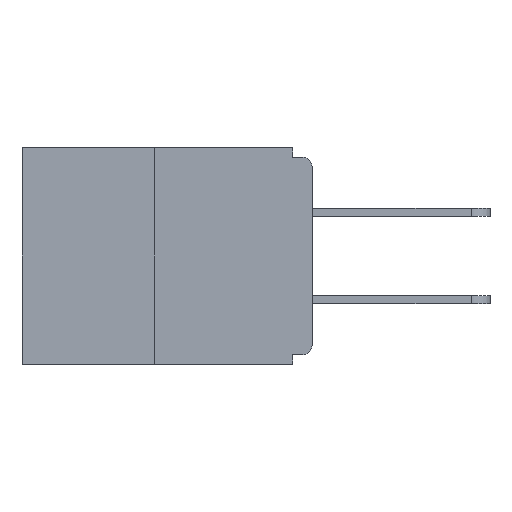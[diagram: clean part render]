
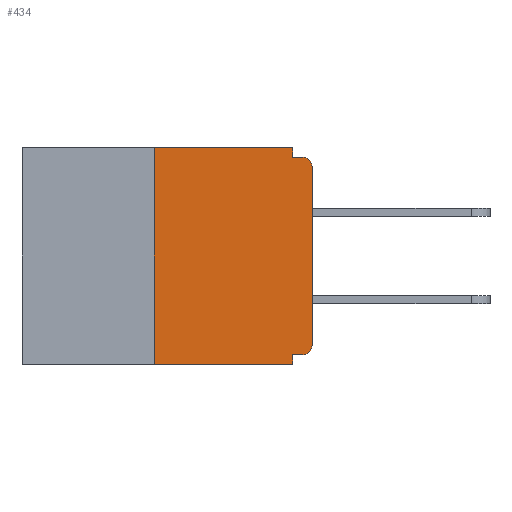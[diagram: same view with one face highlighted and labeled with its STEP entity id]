
A CAD part, left-side view. The second image highlights one B-rep face of the part: STEP entity #434.
In plain terms, the highlighted planar face has unit normal (-1, 0, 0).
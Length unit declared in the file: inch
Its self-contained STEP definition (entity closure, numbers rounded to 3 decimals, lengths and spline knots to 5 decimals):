
#392 = CARTESIAN_POINT ( 'NONE',  ( 0., 0.015, -0.015 ) ) ;
#434 = ADVANCED_FACE ( 'NONE', ( #11077 ), #12126, .F. ) ;
#516 = CARTESIAN_POINT ( 'NONE',  ( 0., 0.46, -0.343 ) ) ;
#550 = DIRECTION ( 'NONE',  ( -1., 0., 0. ) ) ;
#561 = CARTESIAN_POINT ( 'NONE',  ( 0., 0., -0.313 ) ) ;
#722 = CARTESIAN_POINT ( 'NONE',  ( 0., 0., -0.328 ) ) ;
#822 = VERTEX_POINT ( 'NONE', #561 ) ;
#909 = EDGE_CURVE ( 'NONE', #7638, #8690, #3916, .T. ) ;
#922 = CARTESIAN_POINT ( 'NONE',  ( 0., 0., -0.03 ) ) ;
#1101 = CARTESIAN_POINT ( 'NONE',  ( 0., 0.015, -0.328 ) ) ;
#1700 = EDGE_CURVE ( 'NONE', #7556, #10894, #4006, .T. ) ;
#1918 = VERTEX_POINT ( 'NONE', #5938 ) ;
#2105 = EDGE_CURVE ( 'NONE', #7172, #822, #6820, .T. ) ;
#2283 = ORIENTED_EDGE ( 'NONE', *, *, #9506, .F. ) ;
#2381 = ORIENTED_EDGE ( 'NONE', *, *, #909, .F. ) ;
#2509 = EDGE_CURVE ( 'NONE', #10184, #7638, #7995, .T. ) ;
#2531 = CARTESIAN_POINT ( 'NONE',  ( 0., 0.031, -0.343 ) ) ;
#2669 = DIRECTION ( 'NONE',  ( 0., 1., 0. ) ) ;
#2683 = VERTEX_POINT ( 'NONE', #4005 ) ;
#2718 = DIRECTION ( 'NONE',  ( 0., 0., -1. ) ) ;
#2997 = CARTESIAN_POINT ( 'NONE',  ( 0., 0.25, 0. ) ) ;
#3436 = VECTOR ( 'NONE', #7219, 39.37008 ) ;
#3525 = DIRECTION ( 'NONE',  ( 0., 0., 1. ) ) ;
#3538 = LINE ( 'NONE', #2531, #10818 ) ;
#3569 = DIRECTION ( 'NONE',  ( 0., 0., -1. ) ) ;
#3680 = CARTESIAN_POINT ( 'NONE',  ( 0., 0., -0.015 ) ) ;
#3856 = VECTOR ( 'NONE', #3525, 39.37008 ) ;
#3916 = LINE ( 'NONE', #8224, #10313 ) ;
#3985 = LINE ( 'NONE', #8047, #5644 ) ;
#4005 = CARTESIAN_POINT ( 'NONE',  ( 0., 0.031, -0.015 ) ) ;
#4006 = CIRCLE ( 'NONE', #6271, 0.015 ) ;
#4394 = EDGE_CURVE ( 'NONE', #10184, #8232, #5365, .T. ) ;
#4419 = DIRECTION ( 'NONE',  ( 0., -1., 0. ) ) ;
#4447 = EDGE_CURVE ( 'NONE', #7172, #1918, #9519, .T. ) ;
#4490 = DIRECTION ( 'NONE',  ( 0., 0., 1. ) ) ;
#4740 = LINE ( 'NONE', #8037, #12024 ) ;
#4776 = AXIS2_PLACEMENT_3D ( 'NONE', #8966, #550, #9967 ) ;
#4802 = ORIENTED_EDGE ( 'NONE', *, *, #7922, .F. ) ;
#5168 = VECTOR ( 'NONE', #6536, 39.37008 ) ;
#5365 = LINE ( 'NONE', #516, #3436 ) ;
#5521 = DIRECTION ( 'NONE',  ( 1., 0., 0. ) ) ;
#5644 = VECTOR ( 'NONE', #4490, 39.37008 ) ;
#5917 = LINE ( 'NONE', #3680, #5168 ) ;
#5933 = EDGE_CURVE ( 'NONE', #822, #7556, #3985, .T. ) ;
#5938 = CARTESIAN_POINT ( 'NONE',  ( 0., 0.031, -0.328 ) ) ;
#6271 = AXIS2_PLACEMENT_3D ( 'NONE', #7486, #12161, #2718 ) ;
#6536 = DIRECTION ( 'NONE',  ( 0., -1., 0. ) ) ;
#6820 = CIRCLE ( 'NONE', #4776, 0.015 ) ;
#7172 = VERTEX_POINT ( 'NONE', #1101 ) ;
#7200 = DIRECTION ( 'NONE',  ( 0., 0., -1. ) ) ;
#7219 = DIRECTION ( 'NONE',  ( 0., -1., 0. ) ) ;
#7486 = CARTESIAN_POINT ( 'NONE',  ( 0., 0.015, -0.03 ) ) ;
#7556 = VERTEX_POINT ( 'NONE', #922 ) ;
#7638 = VERTEX_POINT ( 'NONE', #2997 ) ;
#7922 = EDGE_CURVE ( 'NONE', #2683, #10894, #5917, .T. ) ;
#7995 = LINE ( 'NONE', #11175, #3856 ) ;
#8037 = CARTESIAN_POINT ( 'NONE',  ( 0., 0.031, 0. ) ) ;
#8047 = CARTESIAN_POINT ( 'NONE',  ( 0., 0., 0. ) ) ;
#8224 = CARTESIAN_POINT ( 'NONE',  ( 0., 0.46, 0. ) ) ;
#8232 = VERTEX_POINT ( 'NONE', #11269 ) ;
#8370 = ORIENTED_EDGE ( 'NONE', *, *, #4394, .T. ) ;
#8690 = VERTEX_POINT ( 'NONE', #12005 ) ;
#8859 = ORIENTED_EDGE ( 'NONE', *, *, #4447, .F. ) ;
#8966 = CARTESIAN_POINT ( 'NONE',  ( 0., 0.015, -0.313 ) ) ;
#9019 = CARTESIAN_POINT ( 'NONE',  ( 0., 0.25, -0.343 ) ) ;
#9294 = ORIENTED_EDGE ( 'NONE', *, *, #2105, .T. ) ;
#9506 = EDGE_CURVE ( 'NONE', #8690, #2683, #4740, .T. ) ;
#9519 = LINE ( 'NONE', #722, #11322 ) ;
#9612 = EDGE_CURVE ( 'NONE', #1918, #8232, #3538, .T. ) ;
#9967 = DIRECTION ( 'NONE',  ( 0., 0., -1. ) ) ;
#10118 = DIRECTION ( 'NONE',  ( 0., 0., -1. ) ) ;
#10160 = CARTESIAN_POINT ( 'NONE',  ( 0., 0.46, 0. ) ) ;
#10161 = AXIS2_PLACEMENT_3D ( 'NONE', #10160, #5521, #3569 ) ;
#10184 = VERTEX_POINT ( 'NONE', #9019 ) ;
#10313 = VECTOR ( 'NONE', #4419, 39.37008 ) ;
#10486 = ORIENTED_EDGE ( 'NONE', *, *, #1700, .T. ) ;
#10818 = VECTOR ( 'NONE', #10118, 39.37008 ) ;
#10894 = VERTEX_POINT ( 'NONE', #392 ) ;
#11077 = FACE_OUTER_BOUND ( 'NONE', #11743, .T. ) ;
#11175 = CARTESIAN_POINT ( 'NONE',  ( 0., 0.25, 0. ) ) ;
#11269 = CARTESIAN_POINT ( 'NONE',  ( 0., 0.031, -0.343 ) ) ;
#11322 = VECTOR ( 'NONE', #2669, 39.37008 ) ;
#11590 = ORIENTED_EDGE ( 'NONE', *, *, #5933, .T. ) ;
#11743 = EDGE_LOOP ( 'NONE', ( #2381, #12085, #8370, #12023, #8859, #9294, #11590, #10486, #4802, #2283 ) ) ;
#12005 = CARTESIAN_POINT ( 'NONE',  ( 0., 0.031, 0. ) ) ;
#12023 = ORIENTED_EDGE ( 'NONE', *, *, #9612, .F. ) ;
#12024 = VECTOR ( 'NONE', #7200, 39.37008 ) ;
#12085 = ORIENTED_EDGE ( 'NONE', *, *, #2509, .F. ) ;
#12126 = PLANE ( 'NONE',  #10161 ) ;
#12161 = DIRECTION ( 'NONE',  ( -1., 0., 0. ) ) ;
